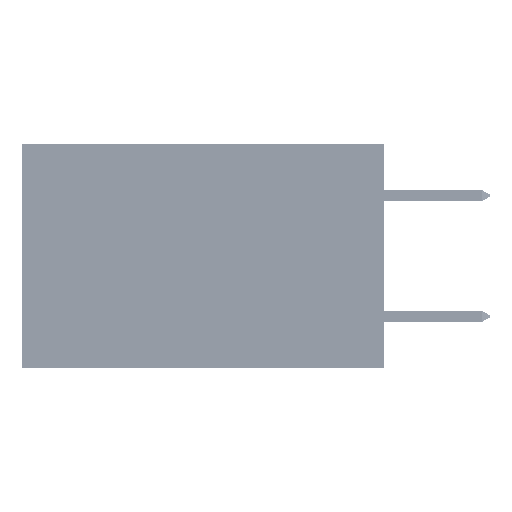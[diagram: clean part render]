
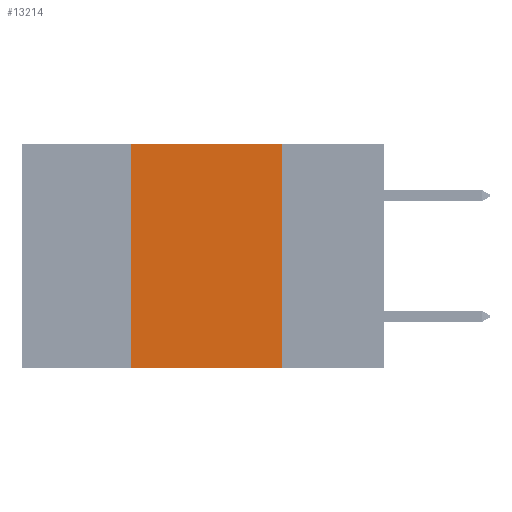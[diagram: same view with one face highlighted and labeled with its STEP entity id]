
A CAD part, left-side view. The second image highlights one B-rep face of the part: STEP entity #13214.
In plain terms, the highlighted planar face has unit normal (-1, 0, 0).
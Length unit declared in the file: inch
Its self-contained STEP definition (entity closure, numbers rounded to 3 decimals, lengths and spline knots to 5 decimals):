
#2954 = CARTESIAN_POINT ( 'NONE',  ( 0., 0.6, -0.37 ) ) ;
#3184 = DIRECTION ( 'NONE',  ( 0., -1., 0. ) ) ;
#5299 = CARTESIAN_POINT ( 'NONE',  ( 0., 0.17, 0. ) ) ;
#7031 = CARTESIAN_POINT ( 'NONE',  ( 0., 0.17, 0. ) ) ;
#8900 = PLANE ( 'NONE',  #23136 ) ;
#10759 = LINE ( 'NONE', #48337, #47251 ) ;
#11955 = ORIENTED_EDGE ( 'NONE', *, *, #22774, .F. ) ;
#13214 = ADVANCED_FACE ( 'NONE', ( #30623 ), #8900, .F. ) ;
#14201 = VECTOR ( 'NONE', #29352, 39.37008 ) ;
#17379 = VERTEX_POINT ( 'NONE', #36684 ) ;
#18615 = VERTEX_POINT ( 'NONE', #22153 ) ;
#20779 = DIRECTION ( 'NONE',  ( 0., 0., 1. ) ) ;
#22153 = CARTESIAN_POINT ( 'NONE',  ( 0., 0.42, -0.37 ) ) ;
#22774 = EDGE_CURVE ( 'NONE', #18615, #24653, #24960, .T. ) ;
#23136 = AXIS2_PLACEMENT_3D ( 'NONE', #35379, #35055, #35540 ) ;
#24220 = VECTOR ( 'NONE', #31515, 39.37008 ) ;
#24380 = CARTESIAN_POINT ( 'NONE',  ( 0., 0.42, 0. ) ) ;
#24653 = VERTEX_POINT ( 'NONE', #36978 ) ;
#24834 = LINE ( 'NONE', #5299, #24220 ) ;
#24960 = LINE ( 'NONE', #24380, #46713 ) ;
#27971 = VERTEX_POINT ( 'NONE', #7031 ) ;
#29352 = DIRECTION ( 'NONE',  ( 0., -1., 0. ) ) ;
#30623 = FACE_OUTER_BOUND ( 'NONE', #32262, .T. ) ;
#31515 = DIRECTION ( 'NONE',  ( 0., 0., -1. ) ) ;
#32262 = EDGE_LOOP ( 'NONE', ( #45956, #47951, #11955, #42066 ) ) ;
#32445 = EDGE_CURVE ( 'NONE', #27971, #17379, #24834, .T. ) ;
#35055 = DIRECTION ( 'NONE',  ( 1., 0., 0. ) ) ;
#35379 = CARTESIAN_POINT ( 'NONE',  ( 0., 0.6, 0. ) ) ;
#35540 = DIRECTION ( 'NONE',  ( 0., 0., -1. ) ) ;
#36684 = CARTESIAN_POINT ( 'NONE',  ( 0., 0.17, -0.37 ) ) ;
#36978 = CARTESIAN_POINT ( 'NONE',  ( 0., 0.42, 0. ) ) ;
#41006 = EDGE_CURVE ( 'NONE', #24653, #27971, #10759, .T. ) ;
#42066 = ORIENTED_EDGE ( 'NONE', *, *, #43588, .T. ) ;
#43588 = EDGE_CURVE ( 'NONE', #18615, #17379, #44183, .T. ) ;
#44183 = LINE ( 'NONE', #2954, #14201 ) ;
#45956 = ORIENTED_EDGE ( 'NONE', *, *, #32445, .F. ) ;
#46713 = VECTOR ( 'NONE', #20779, 39.37008 ) ;
#47251 = VECTOR ( 'NONE', #3184, 39.37008 ) ;
#47951 = ORIENTED_EDGE ( 'NONE', *, *, #41006, .F. ) ;
#48337 = CARTESIAN_POINT ( 'NONE',  ( 0., 0.6, 0. ) ) ;
